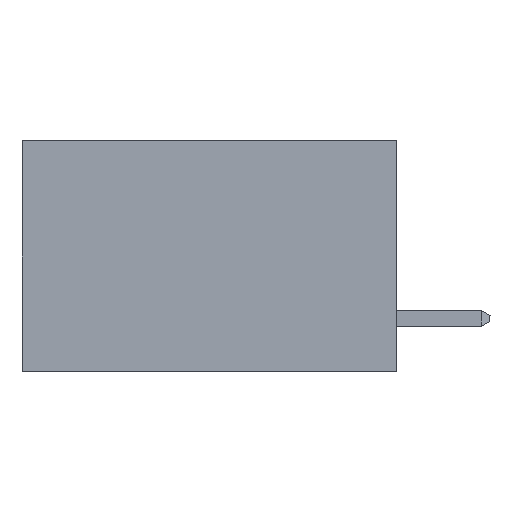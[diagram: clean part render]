
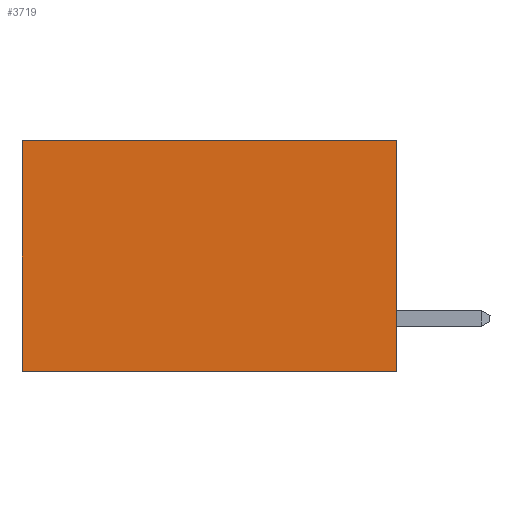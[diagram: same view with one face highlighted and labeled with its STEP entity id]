
A CAD part, left-side view. The second image highlights one B-rep face of the part: STEP entity #3719.
In plain terms, the highlighted planar face has unit normal (-1, 0, 0).
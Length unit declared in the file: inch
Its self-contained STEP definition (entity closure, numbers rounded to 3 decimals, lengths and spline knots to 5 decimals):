
#30 = VECTOR ( 'NONE', #4060, 39.37008 ) ;
#302 = FACE_OUTER_BOUND ( 'NONE', #7737, .T. ) ;
#671 = LINE ( 'NONE', #2377, #5706 ) ;
#911 = PLANE ( 'NONE',  #8080 ) ;
#918 = ORIENTED_EDGE ( 'NONE', *, *, #7305, .T. ) ;
#938 = CARTESIAN_POINT ( 'NONE',  ( 0.2615, 0.6, 0. ) ) ;
#972 = ORIENTED_EDGE ( 'NONE', *, *, #7996, .F. ) ;
#1136 = VERTEX_POINT ( 'NONE', #4540 ) ;
#1289 = VERTEX_POINT ( 'NONE', #938 ) ;
#2167 = LINE ( 'NONE', #9192, #9237 ) ;
#2377 = CARTESIAN_POINT ( 'NONE',  ( 0.2615, 0., -0.37 ) ) ;
#2714 = VERTEX_POINT ( 'NONE', #2934 ) ;
#2909 = CARTESIAN_POINT ( 'NONE',  ( 0.2615, 0.6, -0.37 ) ) ;
#2934 = CARTESIAN_POINT ( 'NONE',  ( 0.2615, 0., 0. ) ) ;
#3020 = DIRECTION ( 'NONE',  ( 0., 0., -1. ) ) ;
#3204 = EDGE_CURVE ( 'NONE', #1289, #4868, #9171, .T. ) ;
#3306 = DIRECTION ( 'NONE',  ( 1., 0., 0. ) ) ;
#3719 = ADVANCED_FACE ( 'NONE', ( #302 ), #911, .F. ) ;
#3898 = VECTOR ( 'NONE', #3020, 39.37008 ) ;
#4060 = DIRECTION ( 'NONE',  ( 0., 1., 0. ) ) ;
#4540 = CARTESIAN_POINT ( 'NONE',  ( 0.2615, 0., -0.37 ) ) ;
#4763 = DIRECTION ( 'NONE',  ( 0., 0., -1. ) ) ;
#4764 = CARTESIAN_POINT ( 'NONE',  ( 0.2615, 0., -0.37 ) ) ;
#4868 = VERTEX_POINT ( 'NONE', #2909 ) ;
#5572 = CARTESIAN_POINT ( 'NONE',  ( 0.2615, 0., -0.37 ) ) ;
#5706 = VECTOR ( 'NONE', #10012, 39.37008 ) ;
#7017 = EDGE_CURVE ( 'NONE', #1136, #4868, #8738, .T. ) ;
#7305 = EDGE_CURVE ( 'NONE', #2714, #1289, #2167, .T. ) ;
#7344 = ORIENTED_EDGE ( 'NONE', *, *, #3204, .T. ) ;
#7662 = CARTESIAN_POINT ( 'NONE',  ( 0.2615, 0.6, -0.37 ) ) ;
#7737 = EDGE_LOOP ( 'NONE', ( #7344, #8728, #972, #918 ) ) ;
#7996 = EDGE_CURVE ( 'NONE', #2714, #1136, #671, .T. ) ;
#8080 = AXIS2_PLACEMENT_3D ( 'NONE', #5572, #3306, #4763 ) ;
#8728 = ORIENTED_EDGE ( 'NONE', *, *, #7017, .F. ) ;
#8738 = LINE ( 'NONE', #4764, #30 ) ;
#9171 = LINE ( 'NONE', #7662, #3898 ) ;
#9192 = CARTESIAN_POINT ( 'NONE',  ( 0.2615, 0., 0. ) ) ;
#9237 = VECTOR ( 'NONE', #10007, 39.37008 ) ;
#10007 = DIRECTION ( 'NONE',  ( 0., 1., 0. ) ) ;
#10012 = DIRECTION ( 'NONE',  ( 0., 0., -1. ) ) ;
